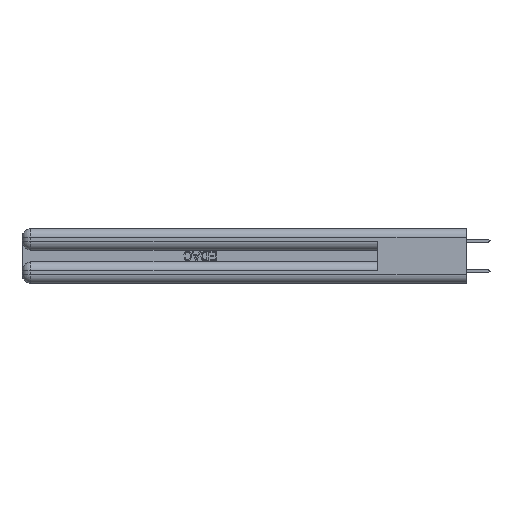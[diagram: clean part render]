
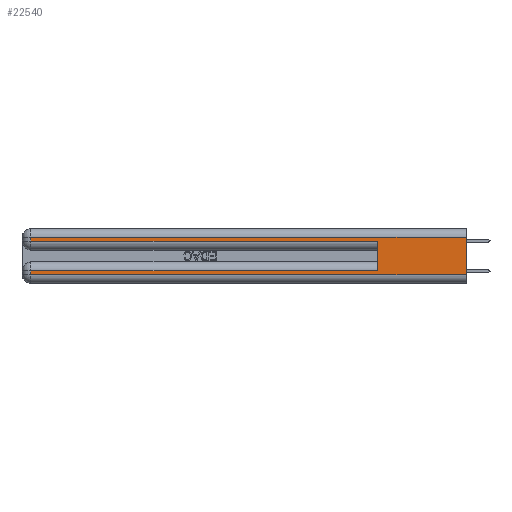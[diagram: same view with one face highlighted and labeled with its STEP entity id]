
A CAD part, left-side view. The second image highlights one B-rep face of the part: STEP entity #22540.
In plain terms, the highlighted planar face has unit normal (-1, 0, 0).
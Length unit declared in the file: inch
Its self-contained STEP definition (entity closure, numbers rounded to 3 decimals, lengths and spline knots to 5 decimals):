
#630 = VERTEX_POINT ( 'NONE', #2970 ) ;
#1288 = EDGE_CURVE ( 'NONE', #13464, #32081, #40013, .T. ) ;
#2255 = DIRECTION ( 'NONE',  ( 1., 0., 0. ) ) ;
#2314 = ORIENTED_EDGE ( 'NONE', *, *, #38817, .F. ) ;
#2585 = VECTOR ( 'NONE', #23070, 39.37008 ) ;
#2970 = CARTESIAN_POINT ( 'NONE',  ( 0., 2.94, 0.31 ) ) ;
#3230 = LINE ( 'NONE', #24817, #23184 ) ;
#3904 = VECTOR ( 'NONE', #32854, 39.37008 ) ;
#4270 = CARTESIAN_POINT ( 'NONE',  ( 0., 2.94, 0.285 ) ) ;
#4447 = ORIENTED_EDGE ( 'NONE', *, *, #25991, .T. ) ;
#4895 = CARTESIAN_POINT ( 'NONE',  ( 0., 0.6, 0.145 ) ) ;
#5042 = CARTESIAN_POINT ( 'NONE',  ( 0., 0.6, 0.285 ) ) ;
#6246 = ORIENTED_EDGE ( 'NONE', *, *, #42482, .F. ) ;
#7554 = DIRECTION ( 'NONE',  ( 0., 1., 0. ) ) ;
#8669 = VECTOR ( 'NONE', #11935, 39.37008 ) ;
#9280 = VECTOR ( 'NONE', #22376, 39.37008 ) ;
#9421 = DIRECTION ( 'NONE',  ( 0., 0., -1. ) ) ;
#9877 = ORIENTED_EDGE ( 'NONE', *, *, #24827, .T. ) ;
#10180 = ORIENTED_EDGE ( 'NONE', *, *, #29833, .T. ) ;
#11490 = CARTESIAN_POINT ( 'NONE',  ( 0., 2.94, 0.085 ) ) ;
#11691 = LINE ( 'NONE', #26730, #2585 ) ;
#11756 = CARTESIAN_POINT ( 'NONE',  ( 0., 0., 0.31 ) ) ;
#11935 = DIRECTION ( 'NONE',  ( 0., 0., -1. ) ) ;
#13464 = VERTEX_POINT ( 'NONE', #4270 ) ;
#13684 = VECTOR ( 'NONE', #23520, 39.37008 ) ;
#14103 = VERTEX_POINT ( 'NONE', #18266 ) ;
#15590 = VECTOR ( 'NONE', #36877, 39.37008 ) ;
#16779 = VECTOR ( 'NONE', #36533, 39.37008 ) ;
#16866 = CARTESIAN_POINT ( 'NONE',  ( 0., 2.94, 0.06 ) ) ;
#18266 = CARTESIAN_POINT ( 'NONE',  ( 0., 0., 0.06 ) ) ;
#20158 = AXIS2_PLACEMENT_3D ( 'NONE', #40473, #2255, #9421 ) ;
#20710 = ORIENTED_EDGE ( 'NONE', *, *, #29969, .T. ) ;
#20885 = ORIENTED_EDGE ( 'NONE', *, *, #1288, .T. ) ;
#22261 = CARTESIAN_POINT ( 'NONE',  ( 0., 2.94, 0.37 ) ) ;
#22376 = DIRECTION ( 'NONE',  ( 0., 0., -1. ) ) ;
#22540 = ADVANCED_FACE ( 'NONE', ( #37101 ), #22913, .F. ) ;
#22913 = PLANE ( 'NONE',  #20158 ) ;
#23070 = DIRECTION ( 'NONE',  ( 0., 0., -1. ) ) ;
#23081 = CARTESIAN_POINT ( 'NONE',  ( 0., 0., 0.06 ) ) ;
#23184 = VECTOR ( 'NONE', #7554, 39.37008 ) ;
#23520 = DIRECTION ( 'NONE',  ( 0., -1., 0. ) ) ;
#24817 = CARTESIAN_POINT ( 'NONE',  ( 0., 0., 0.085 ) ) ;
#24827 = EDGE_CURVE ( 'NONE', #630, #13464, #41174, .T. ) ;
#25479 = CARTESIAN_POINT ( 'NONE',  ( 0., 0., 0.31 ) ) ;
#25991 = EDGE_CURVE ( 'NONE', #34502, #37502, #3230, .T. ) ;
#26730 = CARTESIAN_POINT ( 'NONE',  ( 0., 0., 0.37 ) ) ;
#28391 = VERTEX_POINT ( 'NONE', #16866 ) ;
#28754 = EDGE_CURVE ( 'NONE', #28391, #14103, #29995, .T. ) ;
#29833 = EDGE_CURVE ( 'NONE', #40071, #630, #38078, .T. ) ;
#29969 = EDGE_CURVE ( 'NONE', #37502, #28391, #37026, .T. ) ;
#29995 = LINE ( 'NONE', #23081, #13684 ) ;
#32081 = VERTEX_POINT ( 'NONE', #5042 ) ;
#32514 = EDGE_LOOP ( 'NONE', ( #2314, #10180, #9877, #20885, #6246, #4447, #20710, #43674 ) ) ;
#32854 = DIRECTION ( 'NONE',  ( 0., 1., 0. ) ) ;
#33379 = CARTESIAN_POINT ( 'NONE',  ( 0., 0., 0.285 ) ) ;
#34502 = VERTEX_POINT ( 'NONE', #35969 ) ;
#35969 = CARTESIAN_POINT ( 'NONE',  ( 0., 0.6, 0.085 ) ) ;
#36533 = DIRECTION ( 'NONE',  ( 0., 0., 1. ) ) ;
#36877 = DIRECTION ( 'NONE',  ( 0., -1., 0. ) ) ;
#37026 = LINE ( 'NONE', #39649, #9280 ) ;
#37101 = FACE_OUTER_BOUND ( 'NONE', #32514, .T. ) ;
#37502 = VERTEX_POINT ( 'NONE', #11490 ) ;
#38078 = LINE ( 'NONE', #11756, #3904 ) ;
#38817 = EDGE_CURVE ( 'NONE', #40071, #14103, #11691, .T. ) ;
#39649 = CARTESIAN_POINT ( 'NONE',  ( 0., 2.94, 0.37 ) ) ;
#40013 = LINE ( 'NONE', #33379, #15590 ) ;
#40071 = VERTEX_POINT ( 'NONE', #25479 ) ;
#40473 = CARTESIAN_POINT ( 'NONE',  ( 0., 0., 0.37 ) ) ;
#40664 = LINE ( 'NONE', #4895, #16779 ) ;
#41174 = LINE ( 'NONE', #22261, #8669 ) ;
#42482 = EDGE_CURVE ( 'NONE', #34502, #32081, #40664, .T. ) ;
#43674 = ORIENTED_EDGE ( 'NONE', *, *, #28754, .T. ) ;
